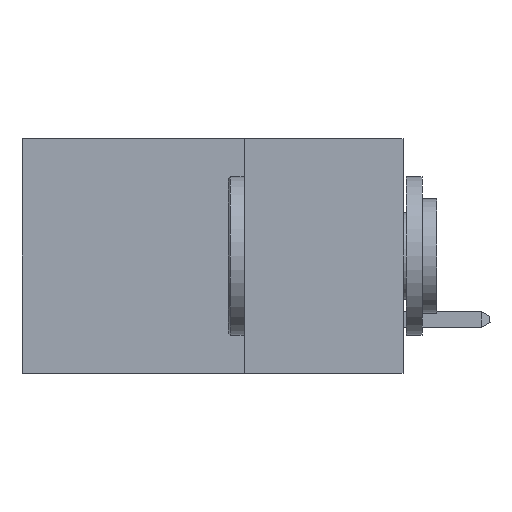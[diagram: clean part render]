
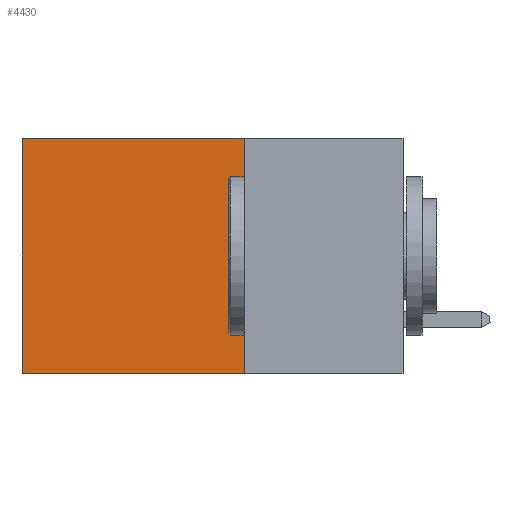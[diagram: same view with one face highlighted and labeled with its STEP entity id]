
A CAD part, left-side view. The second image highlights one B-rep face of the part: STEP entity #4430.
In plain terms, the highlighted planar face has unit normal (-1, 0, 0).
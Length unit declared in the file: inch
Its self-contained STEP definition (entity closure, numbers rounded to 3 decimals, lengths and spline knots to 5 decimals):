
#16 = CARTESIAN_POINT ( 'NONE',  ( 0.2875, 0.25, -0.37 ) ) ;
#154 = DIRECTION ( 'NONE',  ( 0., 1., 0. ) ) ;
#159 = ORIENTED_EDGE ( 'NONE', *, *, #4952, .F. ) ;
#320 = LINE ( 'NONE', #1608, #6343 ) ;
#406 = EDGE_LOOP ( 'NONE', ( #8740, #9519, #159, #1992 ) ) ;
#506 = LINE ( 'NONE', #16, #1831 ) ;
#807 = CARTESIAN_POINT ( 'NONE',  ( 0.2875, 0.25, 0. ) ) ;
#843 = DIRECTION ( 'NONE',  ( 0., 0., -1. ) ) ;
#915 = PLANE ( 'NONE',  #3859 ) ;
#1131 = VERTEX_POINT ( 'NONE', #3616 ) ;
#1608 = CARTESIAN_POINT ( 'NONE',  ( 0.2875, 0.25, 0. ) ) ;
#1831 = VECTOR ( 'NONE', #8433, 39.37008 ) ;
#1929 = CARTESIAN_POINT ( 'NONE',  ( 0.2875, 0.6, 0. ) ) ;
#1992 = ORIENTED_EDGE ( 'NONE', *, *, #3515, .T. ) ;
#2116 = EDGE_CURVE ( 'NONE', #5558, #5641, #9821, .T. ) ;
#2461 = DIRECTION ( 'NONE',  ( 1., 0., 0. ) ) ;
#2466 = VECTOR ( 'NONE', #843, 39.37008 ) ;
#3177 = DIRECTION ( 'NONE',  ( 0., 0., -1. ) ) ;
#3515 = EDGE_CURVE ( 'NONE', #1131, #5558, #320, .T. ) ;
#3565 = CARTESIAN_POINT ( 'NONE',  ( 0.2875, 0.6, -0.37 ) ) ;
#3616 = CARTESIAN_POINT ( 'NONE',  ( 0.2875, 0.25, 0. ) ) ;
#3859 = AXIS2_PLACEMENT_3D ( 'NONE', #3983, #2461, #3177 ) ;
#3983 = CARTESIAN_POINT ( 'NONE',  ( 0.2875, 0.25, 0. ) ) ;
#4136 = VERTEX_POINT ( 'NONE', #9015 ) ;
#4430 = ADVANCED_FACE ( 'NONE', ( #6204 ), #915, .F. ) ;
#4952 = EDGE_CURVE ( 'NONE', #1131, #4136, #5376, .T. ) ;
#5376 = LINE ( 'NONE', #807, #2466 ) ;
#5435 = VECTOR ( 'NONE', #6611, 39.37008 ) ;
#5558 = VERTEX_POINT ( 'NONE', #1929 ) ;
#5641 = VERTEX_POINT ( 'NONE', #3565 ) ;
#5949 = CARTESIAN_POINT ( 'NONE',  ( 0.2875, 0.6, 0. ) ) ;
#6204 = FACE_OUTER_BOUND ( 'NONE', #406, .T. ) ;
#6343 = VECTOR ( 'NONE', #154, 39.37008 ) ;
#6611 = DIRECTION ( 'NONE',  ( 0., 0., -1. ) ) ;
#7414 = EDGE_CURVE ( 'NONE', #4136, #5641, #506, .T. ) ;
#8433 = DIRECTION ( 'NONE',  ( 0., 1., 0. ) ) ;
#8740 = ORIENTED_EDGE ( 'NONE', *, *, #2116, .T. ) ;
#9015 = CARTESIAN_POINT ( 'NONE',  ( 0.2875, 0.25, -0.37 ) ) ;
#9519 = ORIENTED_EDGE ( 'NONE', *, *, #7414, .F. ) ;
#9821 = LINE ( 'NONE', #5949, #5435 ) ;
